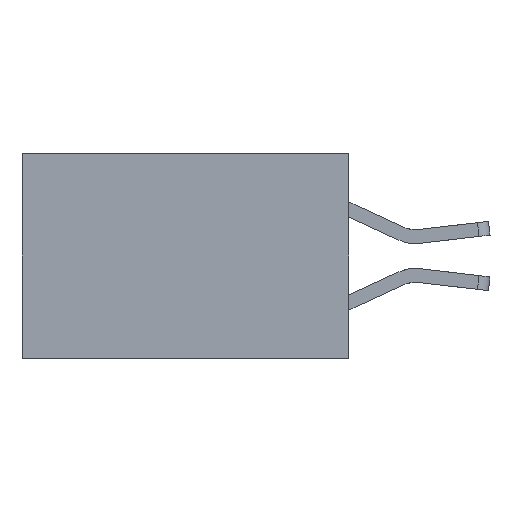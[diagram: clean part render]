
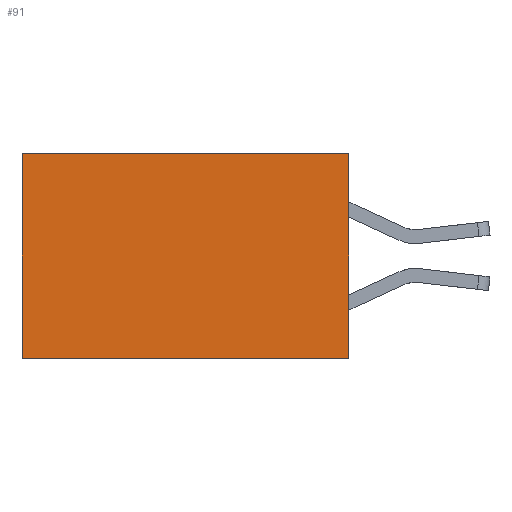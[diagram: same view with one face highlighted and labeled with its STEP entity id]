
A CAD part, left-side view. The second image highlights one B-rep face of the part: STEP entity #91.
In plain terms, the highlighted planar face has unit normal (-1, 0, 0).
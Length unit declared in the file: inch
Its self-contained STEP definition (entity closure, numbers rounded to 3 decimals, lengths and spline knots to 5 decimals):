
#35 = EDGE_CURVE ( 'NONE', #4779, #5033, #247, .T. ) ;
#83 = CARTESIAN_POINT ( 'NONE',  ( 0.277, 0.59, -0.37 ) ) ;
#91 = ADVANCED_FACE ( 'NONE', ( #12466 ), #4681, .F. ) ;
#247 = LINE ( 'NONE', #8750, #5493 ) ;
#336 = CARTESIAN_POINT ( 'NONE',  ( 0.277, 0.59, 0. ) ) ;
#410 = VECTOR ( 'NONE', #9484, 39.37008 ) ;
#1133 = VERTEX_POINT ( 'NONE', #1681 ) ;
#1577 = DIRECTION ( 'NONE',  ( 0., 0., -1. ) ) ;
#1681 = CARTESIAN_POINT ( 'NONE',  ( 0.277, 0.59, -0.37 ) ) ;
#2013 = VERTEX_POINT ( 'NONE', #336 ) ;
#2953 = CARTESIAN_POINT ( 'NONE',  ( 0.277, 0., -0.37 ) ) ;
#3890 = AXIS2_PLACEMENT_3D ( 'NONE', #11649, #12528, #1577 ) ;
#4495 = ORIENTED_EDGE ( 'NONE', *, *, #7308, .F. ) ;
#4681 = PLANE ( 'NONE',  #3890 ) ;
#4779 = VERTEX_POINT ( 'NONE', #12500 ) ;
#5033 = VERTEX_POINT ( 'NONE', #2953 ) ;
#5493 = VECTOR ( 'NONE', #7800, 39.37008 ) ;
#5829 = ORIENTED_EDGE ( 'NONE', *, *, #35, .F. ) ;
#5937 = LINE ( 'NONE', #8473, #410 ) ;
#6835 = VECTOR ( 'NONE', #8024, 39.37008 ) ;
#7055 = LINE ( 'NONE', #83, #12320 ) ;
#7308 = EDGE_CURVE ( 'NONE', #5033, #1133, #9527, .T. ) ;
#7324 = DIRECTION ( 'NONE',  ( 0., 0., -1. ) ) ;
#7800 = DIRECTION ( 'NONE',  ( 0., 0., -1. ) ) ;
#8024 = DIRECTION ( 'NONE',  ( 0., 1., 0. ) ) ;
#8222 = CARTESIAN_POINT ( 'NONE',  ( 0.277, 0., -0.37 ) ) ;
#8473 = CARTESIAN_POINT ( 'NONE',  ( 0.277, 0., 0. ) ) ;
#8513 = EDGE_LOOP ( 'NONE', ( #12186, #4495, #5829, #8902 ) ) ;
#8750 = CARTESIAN_POINT ( 'NONE',  ( 0.277, 0., -0.37 ) ) ;
#8902 = ORIENTED_EDGE ( 'NONE', *, *, #11883, .T. ) ;
#9484 = DIRECTION ( 'NONE',  ( 0., 1., 0. ) ) ;
#9527 = LINE ( 'NONE', #8222, #6835 ) ;
#11649 = CARTESIAN_POINT ( 'NONE',  ( 0.277, 0., -0.37 ) ) ;
#11883 = EDGE_CURVE ( 'NONE', #4779, #2013, #5937, .T. ) ;
#12186 = ORIENTED_EDGE ( 'NONE', *, *, #12394, .T. ) ;
#12320 = VECTOR ( 'NONE', #7324, 39.37008 ) ;
#12394 = EDGE_CURVE ( 'NONE', #2013, #1133, #7055, .T. ) ;
#12466 = FACE_OUTER_BOUND ( 'NONE', #8513, .T. ) ;
#12500 = CARTESIAN_POINT ( 'NONE',  ( 0.277, 0., 0. ) ) ;
#12528 = DIRECTION ( 'NONE',  ( 1., 0., 0. ) ) ;
